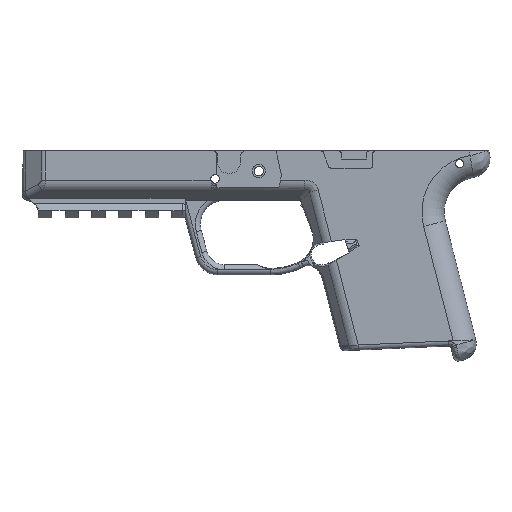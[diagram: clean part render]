
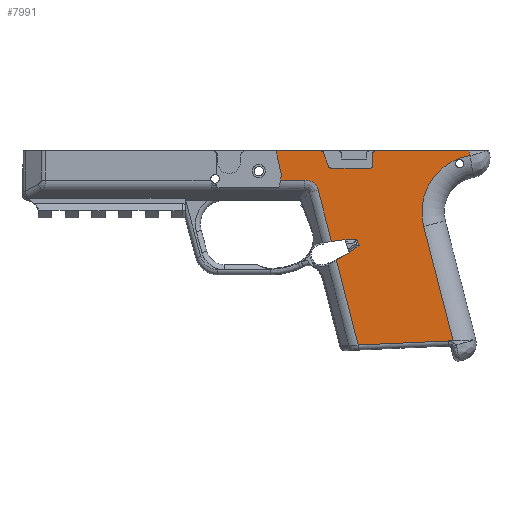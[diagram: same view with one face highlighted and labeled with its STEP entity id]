
A CAD part, left-side view. The second image highlights one B-rep face of the part: STEP entity #7991.
In plain terms, the highlighted face is planar.
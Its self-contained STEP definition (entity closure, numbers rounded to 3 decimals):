
#219=CIRCLE('',#8573,22.475);
#220=CIRCLE('',#8574,7.5);
#221=CIRCLE('',#8575,1.);
#222=CIRCLE('',#8576,1.);
#223=CIRCLE('',#8577,1.);
#224=CIRCLE('',#8578,1.);
#656=FACE_OUTER_BOUND('',#1105,.T.);
#1105=EDGE_LOOP('',(#5995,#5996,#5997,#5998,#5999,#6000,#6001,#6002,#6003,
#6004,#6005,#6006,#6007,#6008,#6009,#6010,#6011,#6012,#6013,#6014,#6015,
#6016,#6017,#6018,#6019,#6020));
#1642=LINE('',#13356,#2388);
#1644=LINE('',#13368,#2390);
#1646=LINE('',#13372,#2392);
#1657=LINE('',#13401,#2403);
#1658=LINE('',#13403,#2404);
#1659=LINE('',#13404,#2405);
#1660=LINE('',#13406,#2406);
#1661=LINE('',#13408,#2407);
#1662=LINE('',#13410,#2408);
#1663=LINE('',#13412,#2409);
#1664=LINE('',#13418,#2410);
#1665=LINE('',#13422,#2411);
#1666=LINE('',#13426,#2412);
#1667=LINE('',#13430,#2413);
#1668=LINE('',#13434,#2414);
#1669=LINE('',#13436,#2415);
#1670=LINE('',#13438,#2416);
#1671=LINE('',#13440,#2417);
#1672=LINE('',#13443,#2418);
#2388=VECTOR('',#9803,10.);
#2390=VECTOR('',#9813,10.);
#2392=VECTOR('',#9817,10.);
#2403=VECTOR('',#9838,10.);
#2404=VECTOR('',#9839,10.);
#2405=VECTOR('',#9840,10.);
#2406=VECTOR('',#9841,10.);
#2407=VECTOR('',#9842,10.);
#2408=VECTOR('',#9843,10.);
#2409=VECTOR('',#9844,10.);
#2410=VECTOR('',#9849,10.);
#2411=VECTOR('',#9852,10.);
#2412=VECTOR('',#9855,10.);
#2413=VECTOR('',#9858,10.);
#2414=VECTOR('',#9861,10.);
#2415=VECTOR('',#9862,10.);
#2416=VECTOR('',#9863,10.);
#2417=VECTOR('',#9864,10.);
#2418=VECTOR('',#9867,10.);
#2962=ELLIPSE('',#8579,10.693,7.);
#3452=VERTEX_POINT('',#13353);
#3453=VERTEX_POINT('',#13355);
#3458=VERTEX_POINT('',#13365);
#3459=VERTEX_POINT('',#13367);
#3460=VERTEX_POINT('',#13371);
#3473=VERTEX_POINT('',#13400);
#3474=VERTEX_POINT('',#13402);
#3475=VERTEX_POINT('',#13405);
#3476=VERTEX_POINT('',#13407);
#3477=VERTEX_POINT('',#13409);
#3478=VERTEX_POINT('',#13411);
#3479=VERTEX_POINT('',#13413);
#3480=VERTEX_POINT('',#13415);
#3481=VERTEX_POINT('',#13417);
#3482=VERTEX_POINT('',#13419);
#3483=VERTEX_POINT('',#13421);
#3484=VERTEX_POINT('',#13423);
#3485=VERTEX_POINT('',#13425);
#3486=VERTEX_POINT('',#13427);
#3487=VERTEX_POINT('',#13429);
#3488=VERTEX_POINT('',#13431);
#3489=VERTEX_POINT('',#13433);
#3490=VERTEX_POINT('',#13435);
#3491=VERTEX_POINT('',#13437);
#3492=VERTEX_POINT('',#13439);
#3493=VERTEX_POINT('',#13441);
#4381=EDGE_CURVE('',#3453,#3452,#1642,.T.);
#4387=EDGE_CURVE('',#3459,#3458,#1644,.T.);
#4389=EDGE_CURVE('',#3460,#3459,#1646,.T.);
#4404=EDGE_CURVE('',#3473,#3458,#1657,.T.);
#4405=EDGE_CURVE('',#3474,#3473,#1658,.T.);
#4406=EDGE_CURVE('',#3453,#3474,#1659,.T.);
#4407=EDGE_CURVE('',#3452,#3475,#1660,.T.);
#4408=EDGE_CURVE('',#3476,#3475,#1661,.T.);
#4409=EDGE_CURVE('',#3477,#3476,#1662,.T.);
#4410=EDGE_CURVE('',#3478,#3477,#1663,.T.);
#4411=EDGE_CURVE('',#3479,#3478,#219,.T.);
#4412=EDGE_CURVE('',#3480,#3479,#220,.T.);
#4413=EDGE_CURVE('',#3480,#3481,#1664,.T.);
#4414=EDGE_CURVE('',#3482,#3481,#221,.T.);
#4415=EDGE_CURVE('',#3482,#3483,#1665,.T.);
#4416=EDGE_CURVE('',#3484,#3483,#222,.T.);
#4417=EDGE_CURVE('',#3484,#3485,#1666,.T.);
#4418=EDGE_CURVE('',#3486,#3485,#223,.T.);
#4419=EDGE_CURVE('',#3487,#3486,#1667,.T.);
#4420=EDGE_CURVE('',#3488,#3487,#224,.T.);
#4421=EDGE_CURVE('',#3489,#3488,#1668,.T.);
#4422=EDGE_CURVE('',#3489,#3490,#1669,.T.);
#4423=EDGE_CURVE('',#3490,#3491,#1670,.T.);
#4424=EDGE_CURVE('',#3492,#3491,#1671,.T.);
#4425=EDGE_CURVE('',#3493,#3492,#2962,.T.);
#4426=EDGE_CURVE('',#3460,#3493,#1672,.T.);
#5995=ORIENTED_EDGE('',*,*,#4387,.T.);
#5996=ORIENTED_EDGE('',*,*,#4404,.F.);
#5997=ORIENTED_EDGE('',*,*,#4405,.F.);
#5998=ORIENTED_EDGE('',*,*,#4406,.F.);
#5999=ORIENTED_EDGE('',*,*,#4381,.T.);
#6000=ORIENTED_EDGE('',*,*,#4407,.T.);
#6001=ORIENTED_EDGE('',*,*,#4408,.F.);
#6002=ORIENTED_EDGE('',*,*,#4409,.F.);
#6003=ORIENTED_EDGE('',*,*,#4410,.F.);
#6004=ORIENTED_EDGE('',*,*,#4411,.F.);
#6005=ORIENTED_EDGE('',*,*,#4412,.F.);
#6006=ORIENTED_EDGE('',*,*,#4413,.T.);
#6007=ORIENTED_EDGE('',*,*,#4414,.F.);
#6008=ORIENTED_EDGE('',*,*,#4415,.T.);
#6009=ORIENTED_EDGE('',*,*,#4416,.F.);
#6010=ORIENTED_EDGE('',*,*,#4417,.T.);
#6011=ORIENTED_EDGE('',*,*,#4418,.F.);
#6012=ORIENTED_EDGE('',*,*,#4419,.F.);
#6013=ORIENTED_EDGE('',*,*,#4420,.F.);
#6014=ORIENTED_EDGE('',*,*,#4421,.F.);
#6015=ORIENTED_EDGE('',*,*,#4422,.T.);
#6016=ORIENTED_EDGE('',*,*,#4423,.T.);
#6017=ORIENTED_EDGE('',*,*,#4424,.F.);
#6018=ORIENTED_EDGE('',*,*,#4425,.F.);
#6019=ORIENTED_EDGE('',*,*,#4426,.F.);
#6020=ORIENTED_EDGE('',*,*,#4389,.T.);
#7681=PLANE('',#8572);
#7991=ADVANCED_FACE('',(#656),#7681,.F.);
#8572=AXIS2_PLACEMENT_3D('',#13399,#9836,#9837);
#8573=AXIS2_PLACEMENT_3D('',#13414,#9845,#9846);
#8574=AXIS2_PLACEMENT_3D('',#13416,#9847,#9848);
#8575=AXIS2_PLACEMENT_3D('',#13420,#9850,#9851);
#8576=AXIS2_PLACEMENT_3D('',#13424,#9853,#9854);
#8577=AXIS2_PLACEMENT_3D('',#13428,#9856,#9857);
#8578=AXIS2_PLACEMENT_3D('',#13432,#9859,#9860);
#8579=AXIS2_PLACEMENT_3D('',#13442,#9865,#9866);
#9803=DIRECTION('',(0.,-0.323,0.947));
#9813=DIRECTION('',(0.,-0.323,0.947));
#9817=DIRECTION('',(0.,-0.991,-0.136));
#9836=DIRECTION('center_axis',(-1.,0.,0.));
#9837=DIRECTION('ref_axis',(0.,1.,0.));
#9838=DIRECTION('',(0.,0.998,0.056));
#9839=DIRECTION('',(0.,0.323,-0.947));
#9840=DIRECTION('',(0.,-0.828,-0.56));
#9841=DIRECTION('',(0.,0.87,0.492));
#9842=DIRECTION('',(0.,0.249,-0.969));
#9843=DIRECTION('',(0.,0.999,0.044));
#9844=DIRECTION('',(0.,-0.249,0.969));
#9845=DIRECTION('center_axis',(1.,0.,0.));
#9846=DIRECTION('ref_axis',(0.,0.,1.));
#9847=DIRECTION('center_axis',(1.,0.,0.));
#9848=DIRECTION('ref_axis',(0.,-0.97,-0.244));
#9849=DIRECTION('',(0.,1.,0.));
#9850=DIRECTION('center_axis',(-1.,0.,0.));
#9851=DIRECTION('ref_axis',(0.,0.707,-0.707));
#9852=DIRECTION('',(0.,0.,1.));
#9853=DIRECTION('center_axis',(1.,0.,0.));
#9854=DIRECTION('ref_axis',(0.,-0.707,0.707));
#9855=DIRECTION('',(0.,1.,0.));
#9856=DIRECTION('center_axis',(1.,0.,0.));
#9857=DIRECTION('ref_axis',(0.,0.576,0.817));
#9858=DIRECTION('',(0.,-0.336,0.942));
#9859=DIRECTION('center_axis',(-1.,0.,0.));
#9860=DIRECTION('ref_axis',(0.,-0.576,-0.817));
#9861=DIRECTION('',(0.,-1.,0.));
#9862=DIRECTION('',(0.,-0.21,0.978));
#9863=DIRECTION('',(0.,0.21,0.978));
#9864=DIRECTION('',(0.,1.,0.));
#9865=DIRECTION('center_axis',(1.,0.,0.));
#9866=DIRECTION('ref_axis',(0.,-0.714,-0.7));
#9867=DIRECTION('',(0.,0.249,-0.969));
#13353=CARTESIAN_POINT('',(22.175,-34.01,32.318));
#13355=CARTESIAN_POINT('',(22.175,-33.995,32.275));
#13356=CARTESIAN_POINT('',(22.175,-27.197,12.322));
#13365=CARTESIAN_POINT('',(22.175,-32.296,27.288));
#13367=CARTESIAN_POINT('',(22.175,-32.284,27.253));
#13368=CARTESIAN_POINT('',(22.175,-27.197,12.322));
#13371=CARTESIAN_POINT('',(22.175,-27.009,27.98));
#13372=CARTESIAN_POINT('',(22.175,-17.622,29.272));
#13399=CARTESIAN_POINT('Origin',(22.175,-7.921,2.186));
#13400=CARTESIAN_POINT('',(22.175,-36.962,27.028));
#13401=CARTESIAN_POINT('',(22.175,-22.893,27.813));
#13402=CARTESIAN_POINT('',(22.175,-37.859,29.661));
#13403=CARTESIAN_POINT('',(22.175,-32.016,12.512));
#13404=CARTESIAN_POINT('',(22.175,-30.049,34.945));
#13405=CARTESIAN_POINT('',(22.175,-28.871,35.225));
#13406=CARTESIAN_POINT('',(22.175,-30.348,34.389));
#13407=CARTESIAN_POINT('',(22.175,-37.447,68.587));
#13408=CARTESIAN_POINT('',(22.175,-26.659,26.619));
#13409=CARTESIAN_POINT('',(22.175,-74.722,66.935));
#13410=CARTESIAN_POINT('',(22.175,-40.785,68.439));
#13411=CARTESIAN_POINT('',(22.175,-63.184,22.049));
#13412=CARTESIAN_POINT('',(22.175,-75.103,68.418));
#13413=CARTESIAN_POINT('',(22.175,-81.332,-5.728));
#13414=CARTESIAN_POINT('Origin',(22.175,-84.951,16.453));
#13415=CARTESIAN_POINT('',(22.175,-81.106,-7.556));
#13416=CARTESIAN_POINT('Origin',(22.175,-88.606,-7.556));
#13417=CARTESIAN_POINT('',(22.175,-44.284,-7.556));
#13418=CARTESIAN_POINT('',(22.175,-84.951,-7.556));
#13419=CARTESIAN_POINT('',(22.175,-43.284,-6.556));
#13420=CARTESIAN_POINT('Origin',(22.175,-44.284,-6.556));
#13421=CARTESIAN_POINT('',(22.175,-43.284,-1.806));
#13422=CARTESIAN_POINT('',(22.175,-43.284,-2.685));
#13423=CARTESIAN_POINT('',(22.175,-42.284,-0.806));
#13424=CARTESIAN_POINT('Origin',(22.175,-42.284,-1.806));
#13425=CARTESIAN_POINT('',(22.175,-26.754,-0.806));
#13426=CARTESIAN_POINT('',(22.175,-30.774,-0.806));
#13427=CARTESIAN_POINT('',(22.175,-25.812,-1.47));
#13428=CARTESIAN_POINT('Origin',(22.175,-26.754,-1.806));
#13429=CARTESIAN_POINT('',(22.175,-23.877,-6.892));
#13430=CARTESIAN_POINT('',(22.175,-23.64,-7.556));
#13431=CARTESIAN_POINT('',(22.175,-22.935,-7.556));
#13432=CARTESIAN_POINT('Origin',(22.175,-22.935,-6.556));
#13433=CARTESIAN_POINT('',(22.175,-5.3,-7.556));
#13434=CARTESIAN_POINT('',(22.175,-8.213,-7.556));
#13435=CARTESIAN_POINT('',(22.175,-7.389,2.186));
#13436=CARTESIAN_POINT('',(22.175,-6.356,-2.63));
#13437=CARTESIAN_POINT('',(22.175,-7.025,3.884));
#13438=CARTESIAN_POINT('',(22.175,-7.4,2.132));
#13439=CARTESIAN_POINT('',(22.175,-16.536,3.884));
#13440=CARTESIAN_POINT('',(22.175,33.814,3.884));
#13441=CARTESIAN_POINT('',(22.175,-21.783,7.651));
#13442=CARTESIAN_POINT('Origin',(22.175,-12.907,12.884));
#13443=CARTESIAN_POINT('',(22.175,-26.659,26.619));
